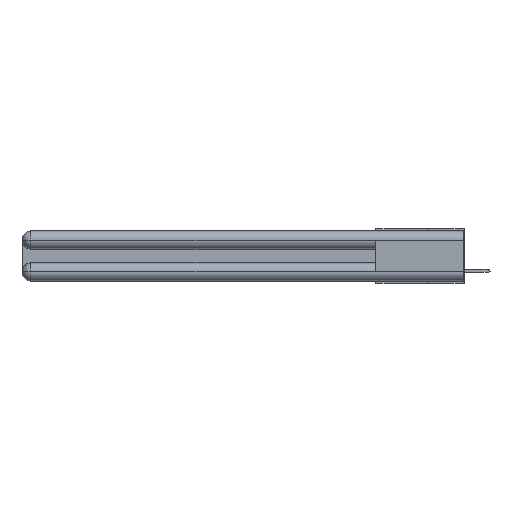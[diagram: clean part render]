
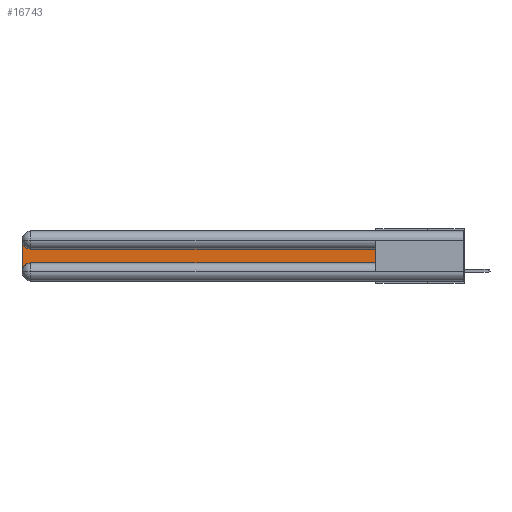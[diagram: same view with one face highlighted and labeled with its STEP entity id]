
A CAD part, left-side view. The second image highlights one B-rep face of the part: STEP entity #16743.
In plain terms, the highlighted planar face has unit normal (-1, 0, 0).
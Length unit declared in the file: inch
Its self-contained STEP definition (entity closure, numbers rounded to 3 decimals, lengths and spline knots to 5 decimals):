
#979 = CARTESIAN_POINT ( 'NONE',  ( 0.075, 3., -0.0625 ) ) ;
#1957 = CIRCLE ( 'NONE', #7743, 0.06 ) ;
#2253 = CARTESIAN_POINT ( 'NONE',  ( 0.075, 0.6, -0.1225 ) ) ;
#2307 = ORIENTED_EDGE ( 'NONE', *, *, #15521, .T. ) ;
#2619 = AXIS2_PLACEMENT_3D ( 'NONE', #26687, #19990, #19879 ) ;
#3752 = DIRECTION ( 'NONE',  ( 0., -1., 0. ) ) ;
#4475 = LINE ( 'NONE', #17565, #9145 ) ;
#4595 = ORIENTED_EDGE ( 'NONE', *, *, #10176, .T. ) ;
#4636 = VECTOR ( 'NONE', #4747, 39.37008 ) ;
#4747 = DIRECTION ( 'NONE',  ( 0., 1., 0. ) ) ;
#5380 = VERTEX_POINT ( 'NONE', #17580 ) ;
#5862 = CARTESIAN_POINT ( 'NONE',  ( 0.075, 3., -0.2175 ) ) ;
#6111 = DIRECTION ( 'NONE',  ( 1., 0., 0. ) ) ;
#6201 = CARTESIAN_POINT ( 'NONE',  ( 0.075, 3., -0.2775 ) ) ;
#7484 = VERTEX_POINT ( 'NONE', #22253 ) ;
#7743 = AXIS2_PLACEMENT_3D ( 'NONE', #27132, #24922, #13458 ) ;
#8053 = VERTEX_POINT ( 'NONE', #6201 ) ;
#9145 = VECTOR ( 'NONE', #3752, 39.37008 ) ;
#10176 = EDGE_CURVE ( 'NONE', #5380, #13290, #19272, .T. ) ;
#10960 = VECTOR ( 'NONE', #15060, 39.37008 ) ;
#12269 = VERTEX_POINT ( 'NONE', #13157 ) ;
#12773 = CARTESIAN_POINT ( 'NONE',  ( 0.075, 2.94, -0.2775 ) ) ;
#12824 = CARTESIAN_POINT ( 'NONE',  ( 0.075, 2.94, -0.1225 ) ) ;
#12919 = ORIENTED_EDGE ( 'NONE', *, *, #24545, .T. ) ;
#12920 = EDGE_CURVE ( 'NONE', #7484, #12269, #4475, .T. ) ;
#12971 = EDGE_CURVE ( 'NONE', #13290, #29578, #1957, .T. ) ;
#13157 = CARTESIAN_POINT ( 'NONE',  ( 0.075, 0.6, -0.2175 ) ) ;
#13290 = VERTEX_POINT ( 'NONE', #12824 ) ;
#13458 = DIRECTION ( 'NONE',  ( 0., 0., -1. ) ) ;
#14673 = EDGE_CURVE ( 'NONE', #8053, #7484, #24080, .T. ) ;
#15060 = DIRECTION ( 'NONE',  ( 0., 0., -1. ) ) ;
#15097 = DIRECTION ( 'NONE',  ( 0., 0., -1. ) ) ;
#15521 = EDGE_CURVE ( 'NONE', #12269, #5380, #25003, .T. ) ;
#16743 = ADVANCED_FACE ( 'NONE', ( #22458 ), #24694, .F. ) ;
#16891 = ORIENTED_EDGE ( 'NONE', *, *, #12971, .T. ) ;
#17054 = LINE ( 'NONE', #5862, #10960 ) ;
#17565 = CARTESIAN_POINT ( 'NONE',  ( 0.075, 0.6, -0.2175 ) ) ;
#17580 = CARTESIAN_POINT ( 'NONE',  ( 0.075, 0.6, -0.1225 ) ) ;
#17918 = AXIS2_PLACEMENT_3D ( 'NONE', #12773, #6111, #15097 ) ;
#19272 = LINE ( 'NONE', #2253, #4636 ) ;
#19879 = DIRECTION ( 'NONE',  ( 0., 0., -1. ) ) ;
#19990 = DIRECTION ( 'NONE',  ( 1., 0., 0. ) ) ;
#20929 = EDGE_LOOP ( 'NONE', ( #4595, #16891, #12919, #22317, #22973, #2307 ) ) ;
#22253 = CARTESIAN_POINT ( 'NONE',  ( 0.075, 2.94, -0.2175 ) ) ;
#22317 = ORIENTED_EDGE ( 'NONE', *, *, #14673, .T. ) ;
#22458 = FACE_OUTER_BOUND ( 'NONE', #20929, .T. ) ;
#22973 = ORIENTED_EDGE ( 'NONE', *, *, #12920, .T. ) ;
#23059 = DIRECTION ( 'NONE',  ( 0., 0., 1. ) ) ;
#23251 = VECTOR ( 'NONE', #23059, 39.37008 ) ;
#23463 = CARTESIAN_POINT ( 'NONE',  ( 0.075, 0.6, -0.2175 ) ) ;
#24080 = CIRCLE ( 'NONE', #17918, 0.06 ) ;
#24545 = EDGE_CURVE ( 'NONE', #29578, #8053, #17054, .T. ) ;
#24694 = PLANE ( 'NONE',  #2619 ) ;
#24922 = DIRECTION ( 'NONE',  ( 1., 0., 0. ) ) ;
#25003 = LINE ( 'NONE', #23463, #23251 ) ;
#26687 = CARTESIAN_POINT ( 'NONE',  ( 0.075, 3., -0.1225 ) ) ;
#27132 = CARTESIAN_POINT ( 'NONE',  ( 0.075, 2.94, -0.0625 ) ) ;
#29578 = VERTEX_POINT ( 'NONE', #979 ) ;
